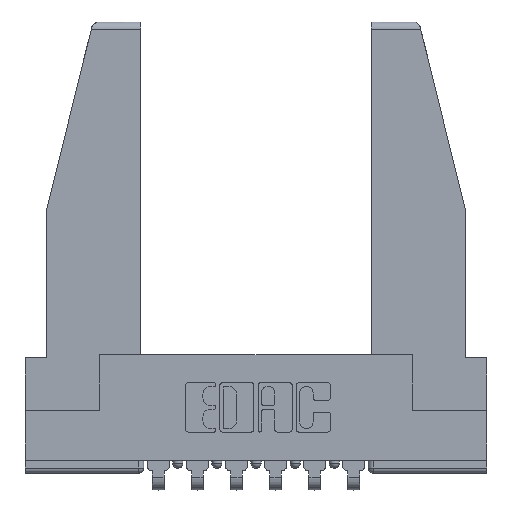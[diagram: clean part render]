
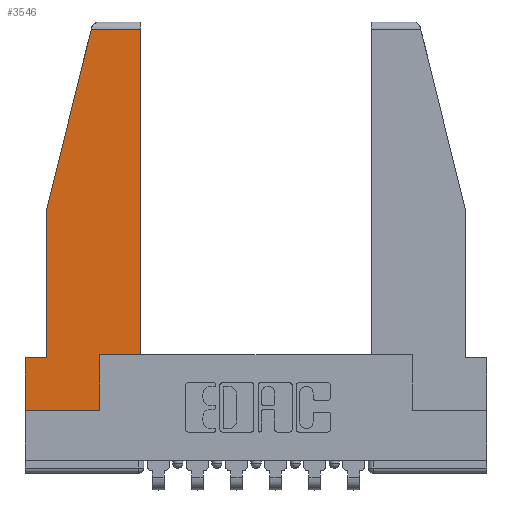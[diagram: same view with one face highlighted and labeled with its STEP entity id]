
A CAD part, top view. The second image highlights one B-rep face of the part: STEP entity #3546.
In plain terms, the highlighted planar face has unit normal (0, 0, 1).
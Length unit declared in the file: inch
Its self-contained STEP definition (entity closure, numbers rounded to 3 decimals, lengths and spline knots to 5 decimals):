
#107 = EDGE_CURVE ( 'NONE', #5534, #10791, #7330, .T. ) ;
#528 = EDGE_CURVE ( 'NONE', #10743, #5615, #6571, .T. ) ;
#559 = ORIENTED_EDGE ( 'NONE', *, *, #1989, .T. ) ;
#670 = VERTEX_POINT ( 'NONE', #2940 ) ;
#1055 = LINE ( 'NONE', #10398, #5913 ) ;
#1074 = EDGE_LOOP ( 'NONE', ( #2096, #559, #1673, #9583, #7498, #4665, #8346, #5618, #7922 ) ) ;
#1401 = VECTOR ( 'NONE', #3922, 39.37008 ) ;
#1673 = ORIENTED_EDGE ( 'NONE', *, *, #11663, .T. ) ;
#1900 = EDGE_CURVE ( 'NONE', #9110, #10743, #1973, .T. ) ;
#1924 = EDGE_CURVE ( 'NONE', #11606, #5534, #1055, .T. ) ;
#1968 = CARTESIAN_POINT ( 'NONE',  ( 0., 0.21, 0. ) ) ;
#1973 = LINE ( 'NONE', #9303, #11793 ) ;
#1989 = EDGE_CURVE ( 'NONE', #5615, #670, #11244, .T. ) ;
#2080 = CARTESIAN_POINT ( 'NONE',  ( 0.297, 0.223, 0. ) ) ;
#2096 = ORIENTED_EDGE ( 'NONE', *, *, #528, .T. ) ;
#2212 = CARTESIAN_POINT ( 'NONE',  ( 0.297, 0., 0. ) ) ;
#2607 = DIRECTION ( 'NONE',  ( -1., 0., 0. ) ) ;
#2711 = PLANE ( 'NONE',  #4777 ) ;
#2940 = CARTESIAN_POINT ( 'NONE',  ( 0.2636, 1.52, 0. ) ) ;
#3017 = LINE ( 'NONE', #11490, #9248 ) ;
#3322 = DIRECTION ( 'NONE',  ( 1., 0., 0. ) ) ;
#3546 = ADVANCED_FACE ( 'NONE', ( #5396 ), #2711, .T. ) ;
#3740 = VECTOR ( 'NONE', #10746, 39.37008 ) ;
#3816 = VECTOR ( 'NONE', #11315, 39.37008 ) ;
#3922 = DIRECTION ( 'NONE',  ( -1., 0., 0. ) ) ;
#3996 = DIRECTION ( 'NONE',  ( 0., -1., 0. ) ) ;
#4269 = CARTESIAN_POINT ( 'NONE',  ( 0.461, 1.52, 0. ) ) ;
#4665 = ORIENTED_EDGE ( 'NONE', *, *, #10350, .T. ) ;
#4777 = AXIS2_PLACEMENT_3D ( 'NONE', #10208, #6260, #11840 ) ;
#5326 = VECTOR ( 'NONE', #10325, 39.37008 ) ;
#5396 = FACE_OUTER_BOUND ( 'NONE', #1074, .T. ) ;
#5534 = VERTEX_POINT ( 'NONE', #10545 ) ;
#5535 = DIRECTION ( 'NONE',  ( 1., 0., 0. ) ) ;
#5615 = VERTEX_POINT ( 'NONE', #4269 ) ;
#5618 = ORIENTED_EDGE ( 'NONE', *, *, #10580, .T. ) ;
#5899 = CARTESIAN_POINT ( 'NONE',  ( 0.271, 1.55, 0. ) ) ;
#5913 = VECTOR ( 'NONE', #12117, 39.37008 ) ;
#6260 = DIRECTION ( 'NONE',  ( 0., 0., 1. ) ) ;
#6571 = LINE ( 'NONE', #8228, #5326 ) ;
#6886 = LINE ( 'NONE', #2212, #3740 ) ;
#6965 = LINE ( 'NONE', #8014, #10719 ) ;
#7241 = EDGE_CURVE ( 'NONE', #11734, #8666, #6965, .T. ) ;
#7330 = LINE ( 'NONE', #12062, #9635 ) ;
#7498 = ORIENTED_EDGE ( 'NONE', *, *, #107, .T. ) ;
#7577 = LINE ( 'NONE', #5899, #3816 ) ;
#7816 = CARTESIAN_POINT ( 'NONE',  ( 0.086, 0.8, 0. ) ) ;
#7922 = ORIENTED_EDGE ( 'NONE', *, *, #1900, .T. ) ;
#8014 = CARTESIAN_POINT ( 'NONE',  ( 0., 0., 0. ) ) ;
#8228 = CARTESIAN_POINT ( 'NONE',  ( 0.461, 0.223, 0. ) ) ;
#8346 = ORIENTED_EDGE ( 'NONE', *, *, #7241, .T. ) ;
#8666 = VERTEX_POINT ( 'NONE', #10419 ) ;
#9110 = VERTEX_POINT ( 'NONE', #2080 ) ;
#9248 = VECTOR ( 'NONE', #3996, 39.37008 ) ;
#9303 = CARTESIAN_POINT ( 'NONE',  ( 0.297, 0.223, 0. ) ) ;
#9583 = ORIENTED_EDGE ( 'NONE', *, *, #1924, .T. ) ;
#9635 = VECTOR ( 'NONE', #2607, 39.37008 ) ;
#9901 = CARTESIAN_POINT ( 'NONE',  ( 0., 0., 0. ) ) ;
#10208 = CARTESIAN_POINT ( 'NONE',  ( 0., 0., 0. ) ) ;
#10325 = DIRECTION ( 'NONE',  ( 0., 1., 0. ) ) ;
#10350 = EDGE_CURVE ( 'NONE', #10791, #11734, #3017, .T. ) ;
#10398 = CARTESIAN_POINT ( 'NONE',  ( 0.086, 0.8, 0. ) ) ;
#10419 = CARTESIAN_POINT ( 'NONE',  ( 0.297, 0., 0. ) ) ;
#10545 = CARTESIAN_POINT ( 'NONE',  ( 0.086, 0.21, 0. ) ) ;
#10580 = EDGE_CURVE ( 'NONE', #8666, #9110, #6886, .T. ) ;
#10719 = VECTOR ( 'NONE', #3322, 39.37008 ) ;
#10743 = VERTEX_POINT ( 'NONE', #11914 ) ;
#10746 = DIRECTION ( 'NONE',  ( 0., 1., 0. ) ) ;
#10791 = VERTEX_POINT ( 'NONE', #1968 ) ;
#11244 = LINE ( 'NONE', #11417, #1401 ) ;
#11315 = DIRECTION ( 'NONE',  ( -0.239, -0.971, 0. ) ) ;
#11417 = CARTESIAN_POINT ( 'NONE',  ( 0., 1.52, 0. ) ) ;
#11490 = CARTESIAN_POINT ( 'NONE',  ( 0., 0.21, 0. ) ) ;
#11606 = VERTEX_POINT ( 'NONE', #7816 ) ;
#11663 = EDGE_CURVE ( 'NONE', #670, #11606, #7577, .T. ) ;
#11734 = VERTEX_POINT ( 'NONE', #9901 ) ;
#11793 = VECTOR ( 'NONE', #5535, 39.37008 ) ;
#11840 = DIRECTION ( 'NONE',  ( 1., 0., 0. ) ) ;
#11914 = CARTESIAN_POINT ( 'NONE',  ( 0.461, 0.223, 0. ) ) ;
#12062 = CARTESIAN_POINT ( 'NONE',  ( 0., 0.21, 0. ) ) ;
#12117 = DIRECTION ( 'NONE',  ( 0., -1., 0. ) ) ;
